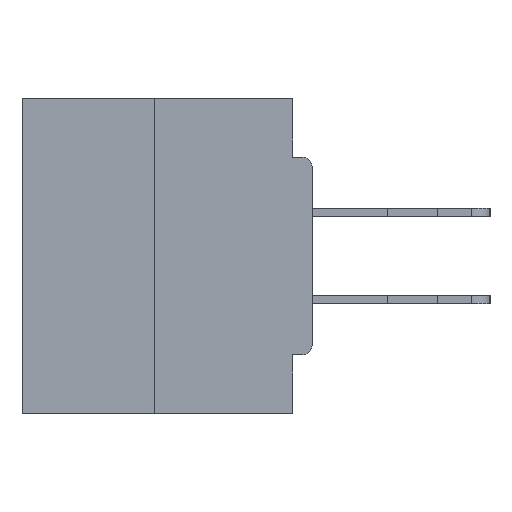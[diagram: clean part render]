
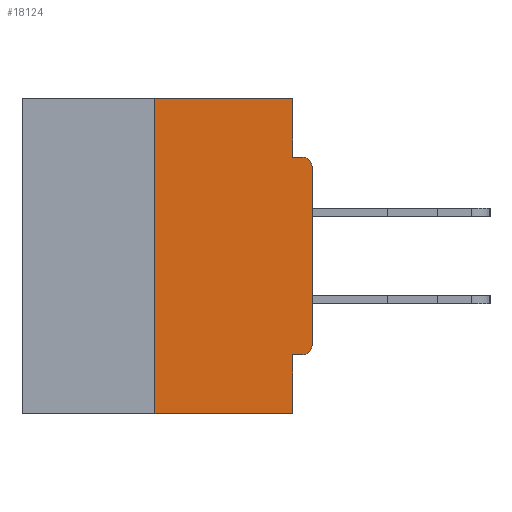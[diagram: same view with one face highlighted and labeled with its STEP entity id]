
A CAD part, left-side view. The second image highlights one B-rep face of the part: STEP entity #18124.
In plain terms, the highlighted planar face has unit normal (-1, 0, 0).
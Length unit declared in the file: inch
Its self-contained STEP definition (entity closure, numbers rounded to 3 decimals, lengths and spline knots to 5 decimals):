
#304 = CARTESIAN_POINT ( 'NONE',  ( 0., 0.46, 0. ) ) ;
#411 = CARTESIAN_POINT ( 'NONE',  ( 0., 0.031, -0.4065 ) ) ;
#670 = DIRECTION ( 'NONE',  ( 0., -1., 0. ) ) ;
#932 = VECTOR ( 'NONE', #670, 39.37008 ) ;
#1767 = EDGE_CURVE ( 'NONE', #22624, #23144, #31440, .T. ) ;
#2101 = DIRECTION ( 'NONE',  ( 0., 0., -1. ) ) ;
#2211 = VECTOR ( 'NONE', #16923, 39.37008 ) ;
#2242 = DIRECTION ( 'NONE',  ( -1., 0., 0. ) ) ;
#2403 = VECTOR ( 'NONE', #20804, 39.37008 ) ;
#2599 = AXIS2_PLACEMENT_3D ( 'NONE', #9857, #2242, #10348 ) ;
#2953 = LINE ( 'NONE', #22923, #19982 ) ;
#3222 = LINE ( 'NONE', #23870, #932 ) ;
#3886 = CARTESIAN_POINT ( 'NONE',  ( 0., 0.25, 0. ) ) ;
#3934 = VECTOR ( 'NONE', #33268, 39.37008 ) ;
#4312 = CARTESIAN_POINT ( 'NONE',  ( 0., 0.031, -0.5 ) ) ;
#5027 = EDGE_CURVE ( 'NONE', #23144, #19026, #12428, .T. ) ;
#6523 = CARTESIAN_POINT ( 'NONE',  ( 0., 0., 0. ) ) ;
#6887 = AXIS2_PLACEMENT_3D ( 'NONE', #27501, #12109, #8890 ) ;
#7582 = FACE_OUTER_BOUND ( 'NONE', #25785, .T. ) ;
#8084 = VERTEX_POINT ( 'NONE', #21398 ) ;
#8369 = EDGE_CURVE ( 'NONE', #22142, #8084, #31246, .T. ) ;
#8890 = DIRECTION ( 'NONE',  ( 0., 0., -1. ) ) ;
#9542 = EDGE_CURVE ( 'NONE', #25855, #29539, #2953, .T. ) ;
#9857 = CARTESIAN_POINT ( 'NONE',  ( 0., 0.015, -0.3915 ) ) ;
#10067 = VECTOR ( 'NONE', #16855, 39.37008 ) ;
#10348 = DIRECTION ( 'NONE',  ( 0., 0., -1. ) ) ;
#11312 = VERTEX_POINT ( 'NONE', #23553 ) ;
#11520 = VECTOR ( 'NONE', #2101, 39.37008 ) ;
#11803 = VERTEX_POINT ( 'NONE', #15073 ) ;
#11938 = LINE ( 'NONE', #6523, #10067 ) ;
#12092 = CARTESIAN_POINT ( 'NONE',  ( 0., 0.031, 0. ) ) ;
#12109 = DIRECTION ( 'NONE',  ( -1., 0., 0. ) ) ;
#12428 = LINE ( 'NONE', #12092, #11520 ) ;
#12542 = EDGE_CURVE ( 'NONE', #8084, #15156, #11938, .T. ) ;
#12684 = CARTESIAN_POINT ( 'NONE',  ( 0., 0.46, -0.5 ) ) ;
#12843 = PLANE ( 'NONE',  #30835 ) ;
#13145 = EDGE_CURVE ( 'NONE', #19026, #11803, #3222, .T. ) ;
#14075 = CARTESIAN_POINT ( 'NONE',  ( 0., 0.031, 0. ) ) ;
#14607 = ORIENTED_EDGE ( 'NONE', *, *, #9542, .F. ) ;
#14732 = VECTOR ( 'NONE', #23009, 39.37008 ) ;
#15073 = CARTESIAN_POINT ( 'NONE',  ( 0., 0.015, -0.0935 ) ) ;
#15156 = VERTEX_POINT ( 'NONE', #18747 ) ;
#16855 = DIRECTION ( 'NONE',  ( 0., 0., 1. ) ) ;
#16923 = DIRECTION ( 'NONE',  ( 0., 0., 1. ) ) ;
#18099 = LINE ( 'NONE', #12684, #14732 ) ;
#18124 = ADVANCED_FACE ( 'NONE', ( #7582 ), #12843, .F. ) ;
#18693 = EDGE_CURVE ( 'NONE', #11312, #22624, #27057, .T. ) ;
#18747 = CARTESIAN_POINT ( 'NONE',  ( 0., 0., -0.1085 ) ) ;
#19026 = VERTEX_POINT ( 'NONE', #21614 ) ;
#19177 = ORIENTED_EDGE ( 'NONE', *, *, #21524, .T. ) ;
#19982 = VECTOR ( 'NONE', #31033, 39.37008 ) ;
#20137 = ORIENTED_EDGE ( 'NONE', *, *, #8369, .T. ) ;
#20152 = ORIENTED_EDGE ( 'NONE', *, *, #5027, .F. ) ;
#20804 = DIRECTION ( 'NONE',  ( 0., -1., 0. ) ) ;
#21398 = CARTESIAN_POINT ( 'NONE',  ( 0., 0., -0.3915 ) ) ;
#21400 = ORIENTED_EDGE ( 'NONE', *, *, #1767, .F. ) ;
#21524 = EDGE_CURVE ( 'NONE', #11312, #29539, #18099, .T. ) ;
#21614 = CARTESIAN_POINT ( 'NONE',  ( 0., 0.031, -0.0935 ) ) ;
#21883 = EDGE_CURVE ( 'NONE', #22142, #25855, #25667, .T. ) ;
#21901 = CARTESIAN_POINT ( 'NONE',  ( 0., 0.25, 0. ) ) ;
#22142 = VERTEX_POINT ( 'NONE', #32064 ) ;
#22624 = VERTEX_POINT ( 'NONE', #21901 ) ;
#22923 = CARTESIAN_POINT ( 'NONE',  ( 0., 0.031, -0.5 ) ) ;
#23009 = DIRECTION ( 'NONE',  ( 0., -1., 0. ) ) ;
#23144 = VERTEX_POINT ( 'NONE', #14075 ) ;
#23163 = DIRECTION ( 'NONE',  ( 1., 0., 0. ) ) ;
#23553 = CARTESIAN_POINT ( 'NONE',  ( 0., 0.25, -0.5 ) ) ;
#23870 = CARTESIAN_POINT ( 'NONE',  ( 0., 0., -0.0935 ) ) ;
#24182 = CARTESIAN_POINT ( 'NONE',  ( 0., 0.46, 0. ) ) ;
#25498 = CARTESIAN_POINT ( 'NONE',  ( 0., 0., -0.4065 ) ) ;
#25619 = EDGE_CURVE ( 'NONE', #15156, #11803, #30139, .T. ) ;
#25667 = LINE ( 'NONE', #25498, #3934 ) ;
#25785 = EDGE_LOOP ( 'NONE', ( #21400, #28039, #19177, #14607, #30920, #20137, #32751, #31028, #32757, #20152 ) ) ;
#25855 = VERTEX_POINT ( 'NONE', #411 ) ;
#27057 = LINE ( 'NONE', #3886, #2211 ) ;
#27501 = CARTESIAN_POINT ( 'NONE',  ( 0., 0.015, -0.1085 ) ) ;
#28039 = ORIENTED_EDGE ( 'NONE', *, *, #18693, .F. ) ;
#28729 = DIRECTION ( 'NONE',  ( 0., 0., -1. ) ) ;
#29539 = VERTEX_POINT ( 'NONE', #4312 ) ;
#30139 = CIRCLE ( 'NONE', #6887, 0.015 ) ;
#30835 = AXIS2_PLACEMENT_3D ( 'NONE', #304, #23163, #28729 ) ;
#30920 = ORIENTED_EDGE ( 'NONE', *, *, #21883, .F. ) ;
#31028 = ORIENTED_EDGE ( 'NONE', *, *, #25619, .T. ) ;
#31033 = DIRECTION ( 'NONE',  ( 0., 0., -1. ) ) ;
#31246 = CIRCLE ( 'NONE', #2599, 0.015 ) ;
#31440 = LINE ( 'NONE', #24182, #2403 ) ;
#32064 = CARTESIAN_POINT ( 'NONE',  ( 0., 0.015, -0.4065 ) ) ;
#32751 = ORIENTED_EDGE ( 'NONE', *, *, #12542, .T. ) ;
#32757 = ORIENTED_EDGE ( 'NONE', *, *, #13145, .F. ) ;
#33268 = DIRECTION ( 'NONE',  ( 0., 1., 0. ) ) ;
